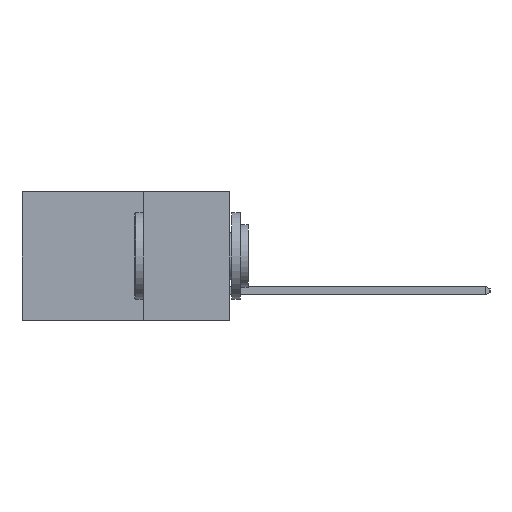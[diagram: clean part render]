
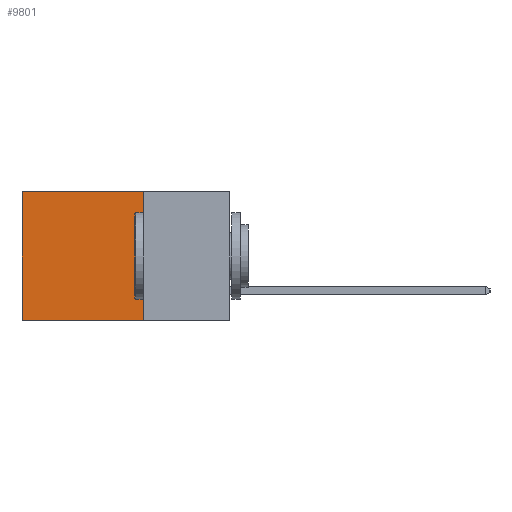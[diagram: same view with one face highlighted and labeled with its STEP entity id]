
A CAD part, left-side view. The second image highlights one B-rep face of the part: STEP entity #9801.
In plain terms, the highlighted planar face has unit normal (-1, 0, 0).
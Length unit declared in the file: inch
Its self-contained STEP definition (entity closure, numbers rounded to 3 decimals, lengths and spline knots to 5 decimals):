
#393 = LINE ( 'NONE', #11418, #8455 ) ;
#560 = VERTEX_POINT ( 'NONE', #8965 ) ;
#733 = EDGE_CURVE ( 'NONE', #7874, #1597, #9944, .T. ) ;
#1552 = DIRECTION ( 'NONE',  ( 0., 0., -1. ) ) ;
#1597 = VERTEX_POINT ( 'NONE', #12639 ) ;
#1784 = DIRECTION ( 'NONE',  ( 0., 0., -1. ) ) ;
#2090 = EDGE_LOOP ( 'NONE', ( #10583, #2445, #5565, #4453 ) ) ;
#2445 = ORIENTED_EDGE ( 'NONE', *, *, #10350, .F. ) ;
#3538 = CARTESIAN_POINT ( 'NONE',  ( 0.2615, 0.25, 0. ) ) ;
#3915 = VECTOR ( 'NONE', #4425, 39.37008 ) ;
#4224 = LINE ( 'NONE', #5418, #3915 ) ;
#4303 = CARTESIAN_POINT ( 'NONE',  ( 0.2615, 0.25, -0.37 ) ) ;
#4425 = DIRECTION ( 'NONE',  ( 0., 1., 0. ) ) ;
#4446 = DIRECTION ( 'NONE',  ( 0., 1., 0. ) ) ;
#4453 = ORIENTED_EDGE ( 'NONE', *, *, #733, .T. ) ;
#4776 = CARTESIAN_POINT ( 'NONE',  ( 0.2615, 0.25, -0.37 ) ) ;
#5288 = DIRECTION ( 'NONE',  ( 0., 0., -1. ) ) ;
#5418 = CARTESIAN_POINT ( 'NONE',  ( 0.2615, 0.25, -0.37 ) ) ;
#5565 = ORIENTED_EDGE ( 'NONE', *, *, #12122, .F. ) ;
#6515 = LINE ( 'NONE', #4303, #11388 ) ;
#6519 = VERTEX_POINT ( 'NONE', #6538 ) ;
#6538 = CARTESIAN_POINT ( 'NONE',  ( 0.2615, 0.25, -0.37 ) ) ;
#7151 = EDGE_CURVE ( 'NONE', #1597, #560, #393, .T. ) ;
#7340 = AXIS2_PLACEMENT_3D ( 'NONE', #4776, #7780, #1784 ) ;
#7780 = DIRECTION ( 'NONE',  ( 1., 0., 0. ) ) ;
#7874 = VERTEX_POINT ( 'NONE', #10707 ) ;
#8455 = VECTOR ( 'NONE', #1552, 39.37008 ) ;
#8965 = CARTESIAN_POINT ( 'NONE',  ( 0.2615, 0.6, -0.37 ) ) ;
#9709 = PLANE ( 'NONE',  #7340 ) ;
#9801 = ADVANCED_FACE ( 'NONE', ( #10857 ), #9709, .F. ) ;
#9944 = LINE ( 'NONE', #3538, #11875 ) ;
#10350 = EDGE_CURVE ( 'NONE', #6519, #560, #4224, .T. ) ;
#10583 = ORIENTED_EDGE ( 'NONE', *, *, #7151, .T. ) ;
#10707 = CARTESIAN_POINT ( 'NONE',  ( 0.2615, 0.25, 0. ) ) ;
#10857 = FACE_OUTER_BOUND ( 'NONE', #2090, .T. ) ;
#11388 = VECTOR ( 'NONE', #5288, 39.37008 ) ;
#11418 = CARTESIAN_POINT ( 'NONE',  ( 0.2615, 0.6, -0.37 ) ) ;
#11875 = VECTOR ( 'NONE', #4446, 39.37008 ) ;
#12122 = EDGE_CURVE ( 'NONE', #7874, #6519, #6515, .T. ) ;
#12639 = CARTESIAN_POINT ( 'NONE',  ( 0.2615, 0.6, 0. ) ) ;
